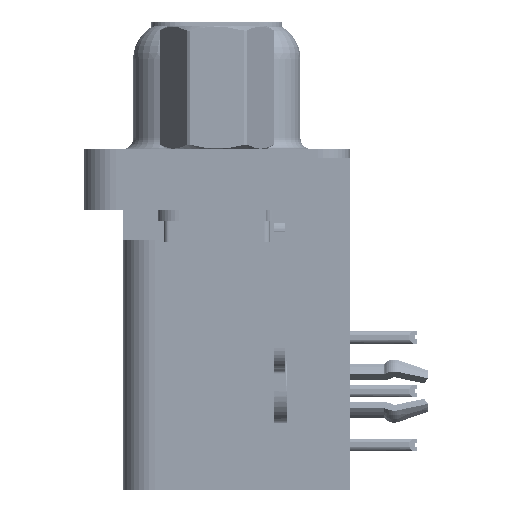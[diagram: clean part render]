
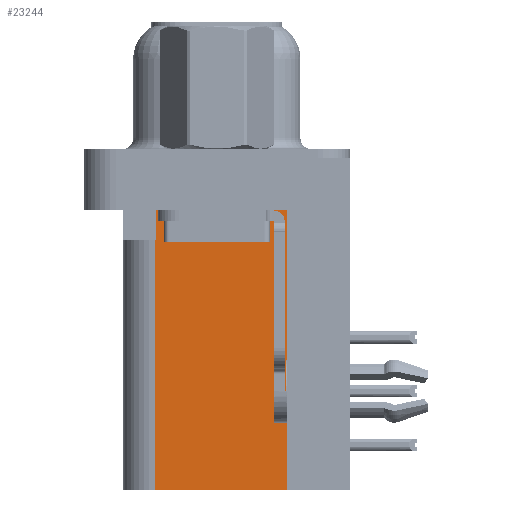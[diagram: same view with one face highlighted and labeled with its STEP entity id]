
A CAD part, left-side view. The second image highlights one B-rep face of the part: STEP entity #23244.
In plain terms, the highlighted planar face has unit normal (-1, 0, 0).
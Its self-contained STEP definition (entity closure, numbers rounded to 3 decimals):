
#2986 = ORIENTED_EDGE ( 'NONE', *, *, #55091, .T. ) ;
#4834 = CARTESIAN_POINT ( 'NONE',  ( 3.79, 2.925, -3.9 ) ) ;
#6068 = DIRECTION ( 'NONE',  ( 0., 0., 1. ) ) ;
#9916 = VECTOR ( 'NONE', #6068, 1000. ) ;
#12020 = ORIENTED_EDGE ( 'NONE', *, *, #20968, .T. ) ;
#12279 = CARTESIAN_POINT ( 'NONE',  ( 3.79, 2.895, -3.9 ) ) ;
#13448 = CARTESIAN_POINT ( 'NONE',  ( 3.79, -3.295, -15.7 ) ) ;
#14089 = ORIENTED_EDGE ( 'NONE', *, *, #26015, .T. ) ;
#14694 = CARTESIAN_POINT ( 'NONE',  ( 3.79, 2.925, -15.7 ) ) ;
#14759 = CARTESIAN_POINT ( 'NONE',  ( 3.79, 2.895, -2.5 ) ) ;
#16440 = DIRECTION ( 'NONE',  ( 0., 1., 0. ) ) ;
#18057 = DIRECTION ( 'NONE',  ( 0., 0., 1. ) ) ;
#18219 = DIRECTION ( 'NONE',  ( 0., 1., 0. ) ) ;
#18804 = VECTOR ( 'NONE', #18219, 1000. ) ;
#19159 = CARTESIAN_POINT ( 'NONE',  ( 3.79, -3.295, -15.7 ) ) ;
#19745 = LINE ( 'NONE', #44611, #31923 ) ;
#20968 = EDGE_CURVE ( 'NONE', #51649, #32865, #19745, .T. ) ;
#21409 = CARTESIAN_POINT ( 'NONE',  ( 3.79, 2.895, -3.9 ) ) ;
#22438 = EDGE_CURVE ( 'NONE', #32865, #36433, #56077, .T. ) ;
#22831 = CARTESIAN_POINT ( 'NONE',  ( 3.79, 0., -3.9 ) ) ;
#23244 = ADVANCED_FACE ( 'NONE', ( #41869 ), #51102, .F. ) ;
#23688 = VERTEX_POINT ( 'NONE', #4834 ) ;
#23758 = DIRECTION ( 'NONE',  ( 1., 0., 0. ) ) ;
#24233 = EDGE_LOOP ( 'NONE', ( #12020, #26468, #2986, #27927, #33637, #14089 ) ) ;
#25509 = AXIS2_PLACEMENT_3D ( 'NONE', #42022, #23758, #55646 ) ;
#25728 = VECTOR ( 'NONE', #18057, 1000. ) ;
#26015 = EDGE_CURVE ( 'NONE', #30878, #51649, #37963, .T. ) ;
#26468 = ORIENTED_EDGE ( 'NONE', *, *, #22438, .T. ) ;
#27199 = VERTEX_POINT ( 'NONE', #14694 ) ;
#27927 = ORIENTED_EDGE ( 'NONE', *, *, #36695, .F. ) ;
#28922 = CARTESIAN_POINT ( 'NONE',  ( 3.79, 2.925, -15.7 ) ) ;
#30878 = VERTEX_POINT ( 'NONE', #19159 ) ;
#31876 = VECTOR ( 'NONE', #57892, 1000. ) ;
#31923 = VECTOR ( 'NONE', #49169, 1000. ) ;
#32865 = VERTEX_POINT ( 'NONE', #14759 ) ;
#33637 = ORIENTED_EDGE ( 'NONE', *, *, #46323, .F. ) ;
#33712 = VECTOR ( 'NONE', #16440, 1000. ) ;
#36433 = VERTEX_POINT ( 'NONE', #12279 ) ;
#36695 = EDGE_CURVE ( 'NONE', #27199, #23688, #58516, .T. ) ;
#37963 = LINE ( 'NONE', #13448, #25728 ) ;
#41869 = FACE_OUTER_BOUND ( 'NONE', #24233, .T. ) ;
#42022 = CARTESIAN_POINT ( 'NONE',  ( 3.79, -3.295, -15.7 ) ) ;
#43920 = CARTESIAN_POINT ( 'NONE',  ( 3.79, -3.295, -15.7 ) ) ;
#44611 = CARTESIAN_POINT ( 'NONE',  ( 3.79, -3.295, -2.5 ) ) ;
#46323 = EDGE_CURVE ( 'NONE', #30878, #27199, #47237, .T. ) ;
#47237 = LINE ( 'NONE', #43920, #33712 ) ;
#49169 = DIRECTION ( 'NONE',  ( 0., 1., 0. ) ) ;
#51102 = PLANE ( 'NONE',  #25509 ) ;
#51649 = VERTEX_POINT ( 'NONE', #55490 ) ;
#55091 = EDGE_CURVE ( 'NONE', #36433, #23688, #55207, .T. ) ;
#55207 = LINE ( 'NONE', #22831, #18804 ) ;
#55490 = CARTESIAN_POINT ( 'NONE',  ( 3.79, -3.295, -2.5 ) ) ;
#55646 = DIRECTION ( 'NONE',  ( 0., 0., -1. ) ) ;
#56077 = LINE ( 'NONE', #21409, #31876 ) ;
#57892 = DIRECTION ( 'NONE',  ( 0., 0., -1. ) ) ;
#58516 = LINE ( 'NONE', #28922, #9916 ) ;
